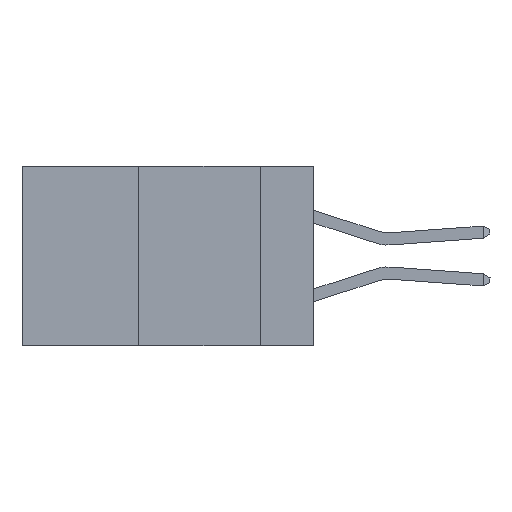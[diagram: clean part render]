
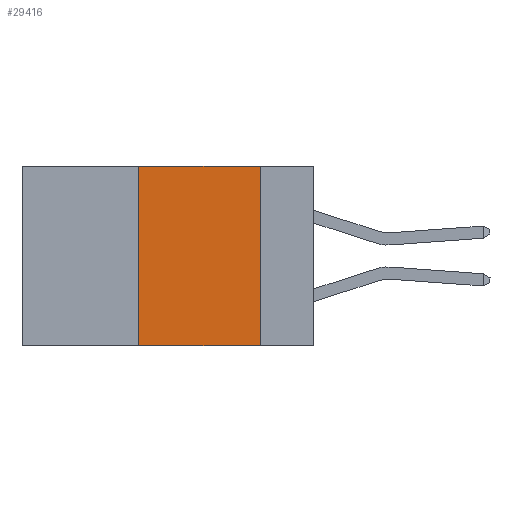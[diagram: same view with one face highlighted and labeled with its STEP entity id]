
A CAD part, left-side view. The second image highlights one B-rep face of the part: STEP entity #29416.
In plain terms, the highlighted planar face has unit normal (-1, 0, 0).
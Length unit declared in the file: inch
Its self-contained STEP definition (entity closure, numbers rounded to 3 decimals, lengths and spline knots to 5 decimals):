
#2208 = LINE ( 'NONE', #20746, #13415 ) ;
#3153 = EDGE_CURVE ( 'NONE', #23401, #41697, #16011, .T. ) ;
#3318 = DIRECTION ( 'NONE',  ( 0., 0., -1. ) ) ;
#3543 = EDGE_LOOP ( 'NONE', ( #39528, #24752, #32899, #16950 ) ) ;
#4783 = VECTOR ( 'NONE', #17869, 39.37008 ) ;
#5278 = VERTEX_POINT ( 'NONE', #33618 ) ;
#6940 = LINE ( 'NONE', #28536, #14046 ) ;
#9078 = DIRECTION ( 'NONE',  ( 0., -1., 0. ) ) ;
#11904 = VERTEX_POINT ( 'NONE', #36578 ) ;
#13415 = VECTOR ( 'NONE', #40399, 39.37008 ) ;
#14046 = VECTOR ( 'NONE', #9078, 39.37008 ) ;
#16011 = LINE ( 'NONE', #22018, #24201 ) ;
#16013 = LINE ( 'NONE', #20858, #4783 ) ;
#16863 = PLANE ( 'NONE',  #33446 ) ;
#16950 = ORIENTED_EDGE ( 'NONE', *, *, #3153, .T. ) ;
#17869 = DIRECTION ( 'NONE',  ( 0., 0., 1. ) ) ;
#20003 = EDGE_CURVE ( 'NONE', #5278, #11904, #6940, .T. ) ;
#20133 = DIRECTION ( 'NONE',  ( 1., 0., 0. ) ) ;
#20746 = CARTESIAN_POINT ( 'NONE',  ( 0., 0.11, 0. ) ) ;
#20858 = CARTESIAN_POINT ( 'NONE',  ( 0., 0.36, 0. ) ) ;
#22018 = CARTESIAN_POINT ( 'NONE',  ( 0., 0.6, -0.37 ) ) ;
#23401 = VERTEX_POINT ( 'NONE', #38934 ) ;
#24201 = VECTOR ( 'NONE', #31721, 39.37008 ) ;
#24523 = EDGE_CURVE ( 'NONE', #23401, #5278, #16013, .T. ) ;
#24752 = ORIENTED_EDGE ( 'NONE', *, *, #20003, .F. ) ;
#25292 = FACE_OUTER_BOUND ( 'NONE', #3543, .T. ) ;
#28536 = CARTESIAN_POINT ( 'NONE',  ( 0., 0.6, 0. ) ) ;
#29416 = ADVANCED_FACE ( 'NONE', ( #25292 ), #16863, .F. ) ;
#31721 = DIRECTION ( 'NONE',  ( 0., -1., 0. ) ) ;
#32845 = CARTESIAN_POINT ( 'NONE',  ( 0., 0.6, 0. ) ) ;
#32899 = ORIENTED_EDGE ( 'NONE', *, *, #24523, .F. ) ;
#33446 = AXIS2_PLACEMENT_3D ( 'NONE', #32845, #20133, #3318 ) ;
#33618 = CARTESIAN_POINT ( 'NONE',  ( 0., 0.36, 0. ) ) ;
#35974 = EDGE_CURVE ( 'NONE', #11904, #41697, #2208, .T. ) ;
#36578 = CARTESIAN_POINT ( 'NONE',  ( 0., 0.11, 0. ) ) ;
#38934 = CARTESIAN_POINT ( 'NONE',  ( 0., 0.36, -0.37 ) ) ;
#39528 = ORIENTED_EDGE ( 'NONE', *, *, #35974, .F. ) ;
#40399 = DIRECTION ( 'NONE',  ( 0., 0., -1. ) ) ;
#41517 = CARTESIAN_POINT ( 'NONE',  ( 0., 0.11, -0.37 ) ) ;
#41697 = VERTEX_POINT ( 'NONE', #41517 ) ;
